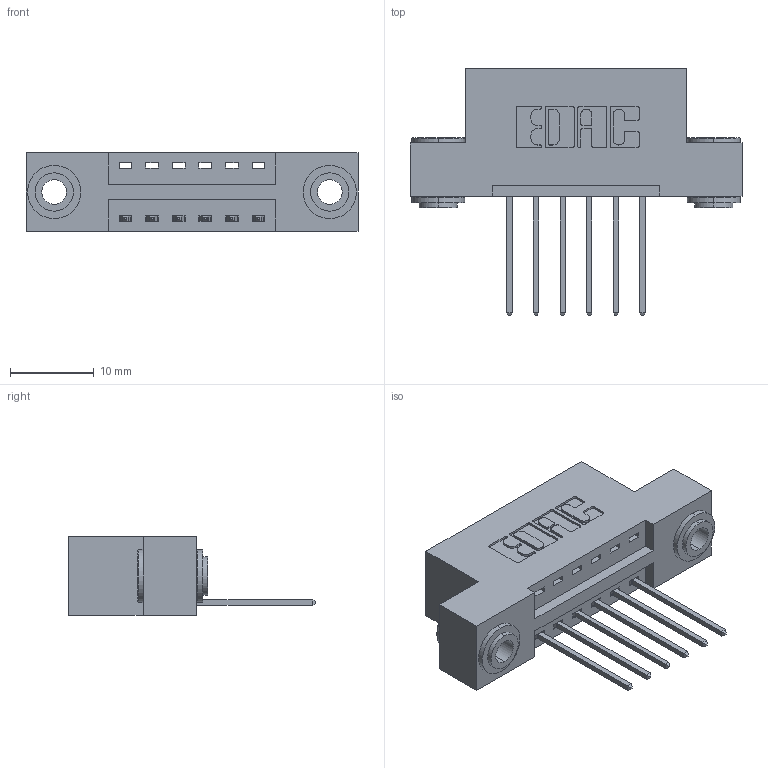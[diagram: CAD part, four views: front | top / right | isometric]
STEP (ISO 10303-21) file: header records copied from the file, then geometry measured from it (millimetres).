
FILE_DESCRIPTION (( 'STEP AP203' ), '1' );
FILE_NAME ('346-006-540-103.STEP', '2022-05-04T18:50:53', ( '' ), ( '' ), 'SwSTEP 2.0', 'SolidWorks 2020', '' );
FILE_SCHEMA (( 'CONFIG_CONTROL_DESIGN' ));
Length unit declared in the file: inch
Products named in the file (4): 345-292-001_345-293-140; 346-006-540-103; 345-250-002_345-250-002-102; 346 Part_Flush Mounting Lugs - 0.156 Dia-TH
Assembly tree (9 placements, depth 2):
  346-006-540-103
    346 Part_Flush Mounting Lugs - 0.156 Dia-TH
    345-292-001_345-293-140  x6
    345-250-002_345-250-002-102  x2
Bounding box: 39.62 x 29.46 x 9.4 mm (x, y, z)
Volume: 3554.3 mm3; surface area: 4364.7 mm2
Topology: 9 solids, 9 shells, 522 faces, 1497 edges, 986 vertices
Faces by surface type: plane 340, cylinder 174, cone 8
Entity records: 9654 total; most frequent: CARTESIAN_POINT 1647, ORIENTED_EDGE 1578, DIRECTION 1527, EDGE_CURVE 789, LINE 609, VECTOR 609, VERTEX_POINT 522, AXIS2_PLACEMENT_3D 459
